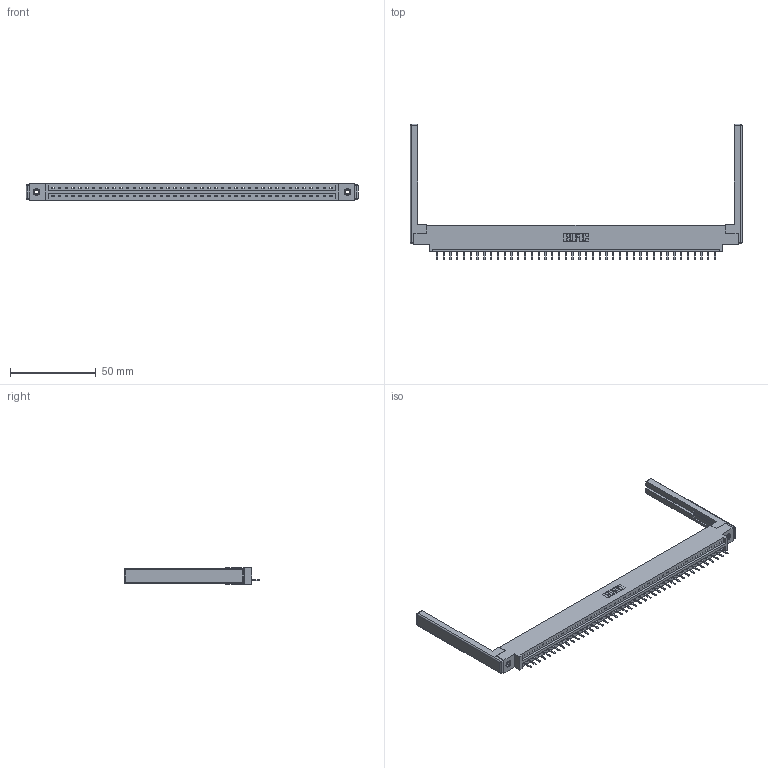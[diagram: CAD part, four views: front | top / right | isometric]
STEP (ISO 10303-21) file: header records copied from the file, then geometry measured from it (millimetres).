
FILE_DESCRIPTION (( 'STEP AP203' ), '1' );
FILE_NAME ('387-042-520-668.STEP', '2019-10-04T20:30:40', ( '' ), ( '' ), 'SwSTEP 2.0', 'SolidWorks 2016', '' );
FILE_SCHEMA (( 'CONFIG_CONTROL_DESIGN' ));
Length unit declared in the file: inch
Products named in the file (5): 387-042-520-668; 345-292-001_345-293-120; 337 Part_0.170 Offset - 0.156 Dia-TI; 307-220-068; 345-250-001_345-250-001-102
Assembly tree (47 placements, depth 2):
  387-042-520-668
    337 Part_0.170 Offset - 0.156 Dia-TI
    345-292-001_345-293-120  x42
    345-250-001_345-250-001-102  x2
    307-220-068  x2
Bounding box: 193.85 x 79.08 x 9.4 mm (x, y, z)
Volume: 24300.6 mm3; surface area: 24327.7 mm2
Topology: 47 solids, 47 shells, 3044 faces, 8945 edges, 5830 vertices
Faces by surface type: plane 2178, cylinder 842, cone 12, sphere 8, torus 4
Entity records: 34226 total; most frequent: CARTESIAN_POINT 5929, ORIENTED_EDGE 5884, DIRECTION 5052, EDGE_CURVE 2942, LINE 2760, VECTOR 2760, VERTEX_POINT 1950, AXIS2_PLACEMENT_3D 1146
